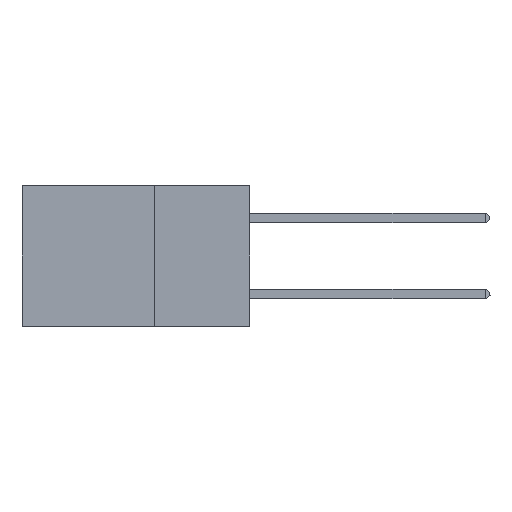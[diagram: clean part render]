
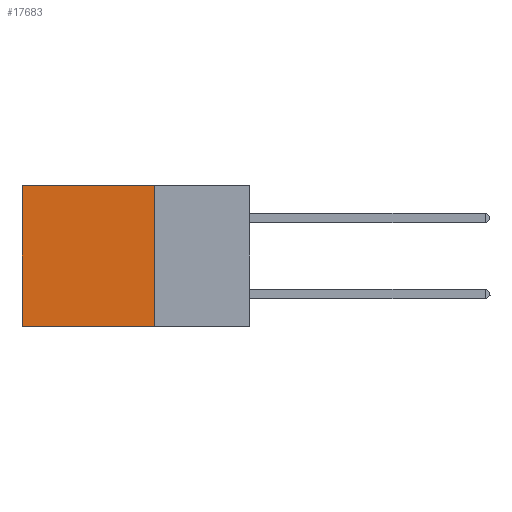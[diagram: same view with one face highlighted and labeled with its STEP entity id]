
A CAD part, left-side view. The second image highlights one B-rep face of the part: STEP entity #17683.
In plain terms, the highlighted planar face has unit normal (-1, 0, 0).
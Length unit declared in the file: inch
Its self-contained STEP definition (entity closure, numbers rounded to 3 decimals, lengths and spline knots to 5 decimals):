
#514 = LINE ( 'NONE', #9869, #13823 ) ;
#1442 = VERTEX_POINT ( 'NONE', #24637 ) ;
#1994 = DIRECTION ( 'NONE',  ( 0., 0., -1. ) ) ;
#2928 = CARTESIAN_POINT ( 'NONE',  ( 0.2875, 0.6, 0. ) ) ;
#4194 = DIRECTION ( 'NONE',  ( 0., 1., 0. ) ) ;
#5805 = EDGE_LOOP ( 'NONE', ( #12730, #10428, #8699, #14479 ) ) ;
#6018 = DIRECTION ( 'NONE',  ( 1., 0., 0. ) ) ;
#8699 = ORIENTED_EDGE ( 'NONE', *, *, #14975, .F. ) ;
#9333 = DIRECTION ( 'NONE',  ( 0., 1., 0. ) ) ;
#9382 = LINE ( 'NONE', #19809, #19257 ) ;
#9869 = CARTESIAN_POINT ( 'NONE',  ( 0.2875, 0.6, 0. ) ) ;
#10428 = ORIENTED_EDGE ( 'NONE', *, *, #12630, .F. ) ;
#10787 = CARTESIAN_POINT ( 'NONE',  ( 0.2875, 0.6, -0.37 ) ) ;
#11675 = VECTOR ( 'NONE', #1994, 39.37008 ) ;
#12139 = VECTOR ( 'NONE', #4194, 39.37008 ) ;
#12423 = CARTESIAN_POINT ( 'NONE',  ( 0.2875, 0.25, 0. ) ) ;
#12587 = EDGE_CURVE ( 'NONE', #27187, #21561, #514, .T. ) ;
#12630 = EDGE_CURVE ( 'NONE', #1442, #21561, #19013, .T. ) ;
#12730 = ORIENTED_EDGE ( 'NONE', *, *, #12587, .T. ) ;
#13823 = VECTOR ( 'NONE', #22650, 39.37008 ) ;
#14479 = ORIENTED_EDGE ( 'NONE', *, *, #22937, .T. ) ;
#14578 = CARTESIAN_POINT ( 'NONE',  ( 0.2875, 0.25, 0. ) ) ;
#14975 = EDGE_CURVE ( 'NONE', #26889, #1442, #15309, .T. ) ;
#15309 = LINE ( 'NONE', #12423, #11675 ) ;
#17122 = FACE_OUTER_BOUND ( 'NONE', #5805, .T. ) ;
#17683 = ADVANCED_FACE ( 'NONE', ( #17122 ), #26848, .F. ) ;
#19013 = LINE ( 'NONE', #27238, #12139 ) ;
#19257 = VECTOR ( 'NONE', #9333, 39.37008 ) ;
#19809 = CARTESIAN_POINT ( 'NONE',  ( 0.2875, 0.25, 0. ) ) ;
#21274 = AXIS2_PLACEMENT_3D ( 'NONE', #14578, #6018, #22894 ) ;
#21561 = VERTEX_POINT ( 'NONE', #10787 ) ;
#22650 = DIRECTION ( 'NONE',  ( 0., 0., -1. ) ) ;
#22894 = DIRECTION ( 'NONE',  ( 0., 0., -1. ) ) ;
#22937 = EDGE_CURVE ( 'NONE', #26889, #27187, #9382, .T. ) ;
#23067 = CARTESIAN_POINT ( 'NONE',  ( 0.2875, 0.25, 0. ) ) ;
#24637 = CARTESIAN_POINT ( 'NONE',  ( 0.2875, 0.25, -0.37 ) ) ;
#26848 = PLANE ( 'NONE',  #21274 ) ;
#26889 = VERTEX_POINT ( 'NONE', #23067 ) ;
#27187 = VERTEX_POINT ( 'NONE', #2928 ) ;
#27238 = CARTESIAN_POINT ( 'NONE',  ( 0.2875, 0.25, -0.37 ) ) ;
